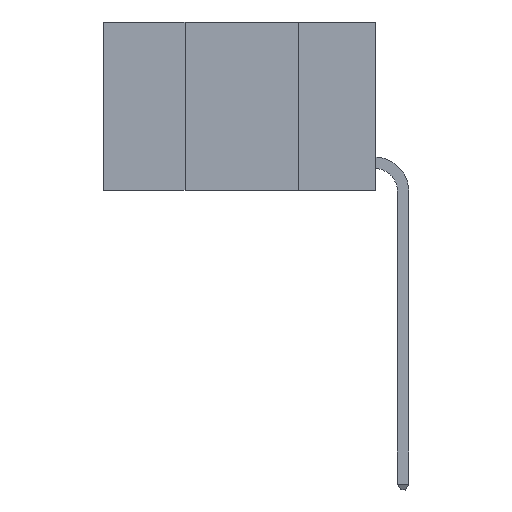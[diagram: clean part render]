
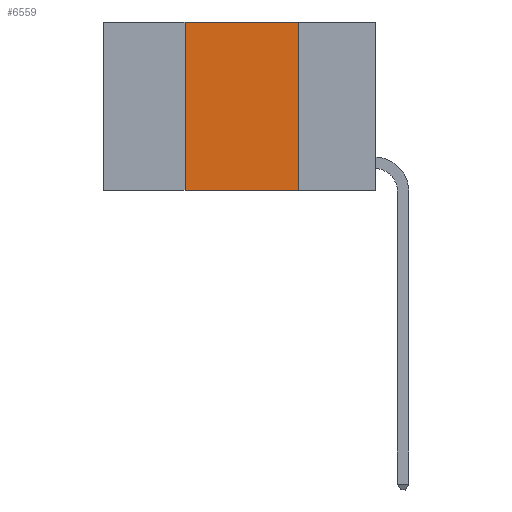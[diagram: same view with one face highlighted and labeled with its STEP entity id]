
A CAD part, left-side view. The second image highlights one B-rep face of the part: STEP entity #6559.
In plain terms, the highlighted planar face has unit normal (-1, 0, 0).
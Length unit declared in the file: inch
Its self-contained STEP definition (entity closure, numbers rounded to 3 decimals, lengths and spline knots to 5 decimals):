
#404 = DIRECTION ( 'NONE',  ( 0., 0., -1. ) ) ;
#973 = CARTESIAN_POINT ( 'NONE',  ( 0., 0.42, -0.37 ) ) ;
#1030 = ORIENTED_EDGE ( 'NONE', *, *, #3837, .F. ) ;
#1242 = FACE_OUTER_BOUND ( 'NONE', #6348, .T. ) ;
#1622 = LINE ( 'NONE', #9178, #11757 ) ;
#1668 = VECTOR ( 'NONE', #16602, 39.37008 ) ;
#1677 = ORIENTED_EDGE ( 'NONE', *, *, #16485, .F. ) ;
#1680 = VERTEX_POINT ( 'NONE', #973 ) ;
#1742 = AXIS2_PLACEMENT_3D ( 'NONE', #16846, #8718, #404 ) ;
#1872 = LINE ( 'NONE', #15301, #8791 ) ;
#2679 = VERTEX_POINT ( 'NONE', #11318 ) ;
#3837 = EDGE_CURVE ( 'NONE', #4314, #4194, #1622, .T. ) ;
#4194 = VERTEX_POINT ( 'NONE', #15418 ) ;
#4314 = VERTEX_POINT ( 'NONE', #15637 ) ;
#6348 = EDGE_LOOP ( 'NONE', ( #1677, #1030, #9359, #15397 ) ) ;
#6559 = ADVANCED_FACE ( 'NONE', ( #1242 ), #7364, .F. ) ;
#6940 = EDGE_CURVE ( 'NONE', #1680, #4314, #9441, .T. ) ;
#7364 = PLANE ( 'NONE',  #1742 ) ;
#7548 = DIRECTION ( 'NONE',  ( 0., 0., -1. ) ) ;
#7887 = DIRECTION ( 'NONE',  ( 0., -1., 0. ) ) ;
#8718 = DIRECTION ( 'NONE',  ( 1., 0., 0. ) ) ;
#8791 = VECTOR ( 'NONE', #16639, 39.37008 ) ;
#9178 = CARTESIAN_POINT ( 'NONE',  ( 0., 0.6, 0. ) ) ;
#9359 = ORIENTED_EDGE ( 'NONE', *, *, #6940, .F. ) ;
#9441 = LINE ( 'NONE', #15259, #1668 ) ;
#11240 = EDGE_CURVE ( 'NONE', #1680, #2679, #1872, .T. ) ;
#11318 = CARTESIAN_POINT ( 'NONE',  ( 0., 0.17, -0.37 ) ) ;
#11757 = VECTOR ( 'NONE', #7887, 39.37008 ) ;
#12041 = VECTOR ( 'NONE', #7548, 39.37008 ) ;
#15259 = CARTESIAN_POINT ( 'NONE',  ( 0., 0.42, 0. ) ) ;
#15301 = CARTESIAN_POINT ( 'NONE',  ( 0., 0.6, -0.37 ) ) ;
#15397 = ORIENTED_EDGE ( 'NONE', *, *, #11240, .T. ) ;
#15418 = CARTESIAN_POINT ( 'NONE',  ( 0., 0.17, 0. ) ) ;
#15636 = LINE ( 'NONE', #16855, #12041 ) ;
#15637 = CARTESIAN_POINT ( 'NONE',  ( 0., 0.42, 0. ) ) ;
#16485 = EDGE_CURVE ( 'NONE', #4194, #2679, #15636, .T. ) ;
#16602 = DIRECTION ( 'NONE',  ( 0., 0., 1. ) ) ;
#16639 = DIRECTION ( 'NONE',  ( 0., -1., 0. ) ) ;
#16846 = CARTESIAN_POINT ( 'NONE',  ( 0., 0.6, 0. ) ) ;
#16855 = CARTESIAN_POINT ( 'NONE',  ( 0., 0.17, 0. ) ) ;
